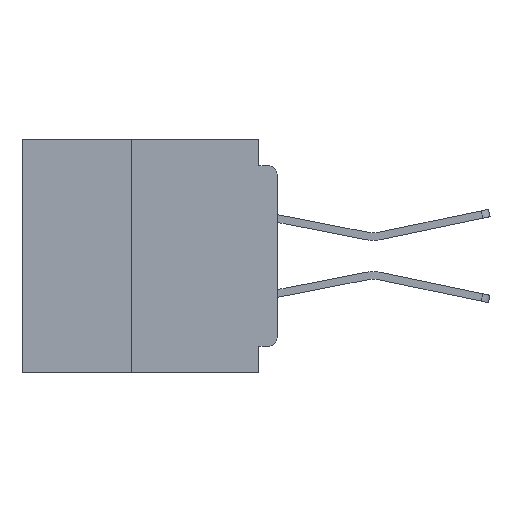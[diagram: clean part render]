
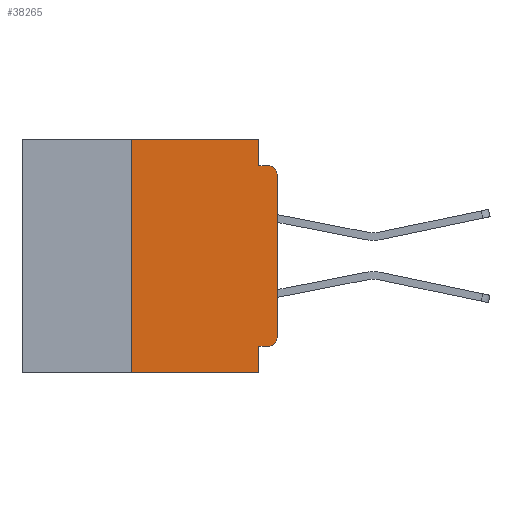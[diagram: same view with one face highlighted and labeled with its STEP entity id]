
A CAD part, left-side view. The second image highlights one B-rep face of the part: STEP entity #38265.
In plain terms, the highlighted planar face has unit normal (-1, 0, 0).
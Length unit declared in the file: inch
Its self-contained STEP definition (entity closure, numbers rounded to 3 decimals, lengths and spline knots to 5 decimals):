
#927 = VERTEX_POINT ( 'NONE', #49150 ) ;
#992 = CARTESIAN_POINT ( 'NONE',  ( 0., 0.031, 0. ) ) ;
#1342 = CARTESIAN_POINT ( 'NONE',  ( 0., 0.437, 0. ) ) ;
#1372 = DIRECTION ( 'NONE',  ( 0., 1., 0. ) ) ;
#1440 = AXIS2_PLACEMENT_3D ( 'NONE', #29363, #5869, #33343 ) ;
#3696 = ORIENTED_EDGE ( 'NONE', *, *, #12835, .F. ) ;
#3741 = VERTEX_POINT ( 'NONE', #19964 ) ;
#4817 = DIRECTION ( 'NONE',  ( 0., 0., -1. ) ) ;
#5144 = AXIS2_PLACEMENT_3D ( 'NONE', #1342, #17262, #44652 ) ;
#5185 = FACE_OUTER_BOUND ( 'NONE', #9568, .T. ) ;
#5342 = PLANE ( 'NONE',  #5144 ) ;
#5869 = DIRECTION ( 'NONE',  ( -1., 0., 0. ) ) ;
#7976 = VERTEX_POINT ( 'NONE', #28218 ) ;
#8350 = LINE ( 'NONE', #8853, #20083 ) ;
#8853 = CARTESIAN_POINT ( 'NONE',  ( 0., 0.437, 0. ) ) ;
#9358 = ORIENTED_EDGE ( 'NONE', *, *, #37518, .F. ) ;
#9568 = EDGE_LOOP ( 'NONE', ( #43590, #33028, #42352, #26870, #9358, #3696, #36937, #41972, #49599, #25554 ) ) ;
#10916 = CARTESIAN_POINT ( 'NONE',  ( 0., 0.015, -0.06 ) ) ;
#11592 = DIRECTION ( 'NONE',  ( 0., -1., 0. ) ) ;
#12835 = EDGE_CURVE ( 'NONE', #27072, #26762, #17643, .T. ) ;
#12872 = EDGE_CURVE ( 'NONE', #3741, #50868, #45205, .T. ) ;
#12972 = CARTESIAN_POINT ( 'NONE',  ( 0., 0.25, -0.4 ) ) ;
#14123 = CIRCLE ( 'NONE', #27518, 0.015 ) ;
#14882 = DIRECTION ( 'NONE',  ( 0., 0., -1. ) ) ;
#15733 = EDGE_CURVE ( 'NONE', #7976, #48995, #24651, .T. ) ;
#16742 = EDGE_CURVE ( 'NONE', #48995, #21191, #50946, .T. ) ;
#16953 = DIRECTION ( 'NONE',  ( 0., 0., 1. ) ) ;
#17242 = EDGE_CURVE ( 'NONE', #927, #21191, #14123, .T. ) ;
#17262 = DIRECTION ( 'NONE',  ( 1., 0., 0. ) ) ;
#17643 = LINE ( 'NONE', #12972, #47654 ) ;
#17782 = CARTESIAN_POINT ( 'NONE',  ( 0., 0., -0.34 ) ) ;
#18326 = DIRECTION ( 'NONE',  ( 0., 0., 1. ) ) ;
#18875 = DIRECTION ( 'NONE',  ( 0., -1., 0. ) ) ;
#19683 = VECTOR ( 'NONE', #18875, 39.37008 ) ;
#19964 = CARTESIAN_POINT ( 'NONE',  ( 0., 0.015, -0.355 ) ) ;
#20083 = VECTOR ( 'NONE', #20740, 39.37008 ) ;
#20740 = DIRECTION ( 'NONE',  ( 0., -1., 0. ) ) ;
#21191 = VERTEX_POINT ( 'NONE', #28040 ) ;
#23510 = CARTESIAN_POINT ( 'NONE',  ( 0., 0.25, -0.4 ) ) ;
#24399 = EDGE_CURVE ( 'NONE', #50927, #927, #27913, .T. ) ;
#24632 = VERTEX_POINT ( 'NONE', #35062 ) ;
#24651 = LINE ( 'NONE', #992, #33835 ) ;
#24898 = CARTESIAN_POINT ( 'NONE',  ( 0., 0.25, 0. ) ) ;
#25554 = ORIENTED_EDGE ( 'NONE', *, *, #26263, .T. ) ;
#26263 = EDGE_CURVE ( 'NONE', #3741, #50927, #36421, .T. ) ;
#26762 = VERTEX_POINT ( 'NONE', #24898 ) ;
#26870 = ORIENTED_EDGE ( 'NONE', *, *, #15733, .F. ) ;
#27072 = VERTEX_POINT ( 'NONE', #23510 ) ;
#27518 = AXIS2_PLACEMENT_3D ( 'NONE', #10916, #38366, #14882 ) ;
#27913 = LINE ( 'NONE', #41791, #38396 ) ;
#28040 = CARTESIAN_POINT ( 'NONE',  ( 0., 0.015, -0.045 ) ) ;
#28218 = CARTESIAN_POINT ( 'NONE',  ( 0., 0.031, 0. ) ) ;
#29363 = CARTESIAN_POINT ( 'NONE',  ( 0., 0.015, -0.34 ) ) ;
#32472 = DIRECTION ( 'NONE',  ( 0., 0., -1. ) ) ;
#33012 = CARTESIAN_POINT ( 'NONE',  ( 0., 0.031, -0.355 ) ) ;
#33028 = ORIENTED_EDGE ( 'NONE', *, *, #17242, .T. ) ;
#33161 = LINE ( 'NONE', #36222, #41169 ) ;
#33343 = DIRECTION ( 'NONE',  ( 0., 0., -1. ) ) ;
#33835 = VECTOR ( 'NONE', #32472, 39.37008 ) ;
#34292 = VECTOR ( 'NONE', #11592, 39.37008 ) ;
#34776 = VECTOR ( 'NONE', #1372, 39.37008 ) ;
#35062 = CARTESIAN_POINT ( 'NONE',  ( 0., 0.031, -0.4 ) ) ;
#36116 = EDGE_CURVE ( 'NONE', #27072, #24632, #45957, .T. ) ;
#36222 = CARTESIAN_POINT ( 'NONE',  ( 0., 0.031, -0.4 ) ) ;
#36421 = CIRCLE ( 'NONE', #1440, 0.015 ) ;
#36937 = ORIENTED_EDGE ( 'NONE', *, *, #36116, .T. ) ;
#37518 = EDGE_CURVE ( 'NONE', #26762, #7976, #8350, .T. ) ;
#38265 = ADVANCED_FACE ( 'NONE', ( #5185 ), #5342, .F. ) ;
#38366 = DIRECTION ( 'NONE',  ( -1., 0., 0. ) ) ;
#38396 = VECTOR ( 'NONE', #18326, 39.37008 ) ;
#38399 = CARTESIAN_POINT ( 'NONE',  ( 0., 0., -0.045 ) ) ;
#40595 = CARTESIAN_POINT ( 'NONE',  ( 0., 0., -0.355 ) ) ;
#41169 = VECTOR ( 'NONE', #4817, 39.37008 ) ;
#41791 = CARTESIAN_POINT ( 'NONE',  ( 0., 0., 0. ) ) ;
#41972 = ORIENTED_EDGE ( 'NONE', *, *, #46323, .F. ) ;
#42352 = ORIENTED_EDGE ( 'NONE', *, *, #16742, .F. ) ;
#43590 = ORIENTED_EDGE ( 'NONE', *, *, #24399, .T. ) ;
#44507 = CARTESIAN_POINT ( 'NONE',  ( 0., 0.031, -0.045 ) ) ;
#44652 = DIRECTION ( 'NONE',  ( 0., 0., -1. ) ) ;
#45205 = LINE ( 'NONE', #40595, #34776 ) ;
#45957 = LINE ( 'NONE', #50863, #34292 ) ;
#46323 = EDGE_CURVE ( 'NONE', #50868, #24632, #33161, .T. ) ;
#47654 = VECTOR ( 'NONE', #16953, 39.37008 ) ;
#48995 = VERTEX_POINT ( 'NONE', #44507 ) ;
#49150 = CARTESIAN_POINT ( 'NONE',  ( 0., 0., -0.06 ) ) ;
#49599 = ORIENTED_EDGE ( 'NONE', *, *, #12872, .F. ) ;
#50863 = CARTESIAN_POINT ( 'NONE',  ( 0., 0.437, -0.4 ) ) ;
#50868 = VERTEX_POINT ( 'NONE', #33012 ) ;
#50927 = VERTEX_POINT ( 'NONE', #17782 ) ;
#50946 = LINE ( 'NONE', #38399, #19683 ) ;
